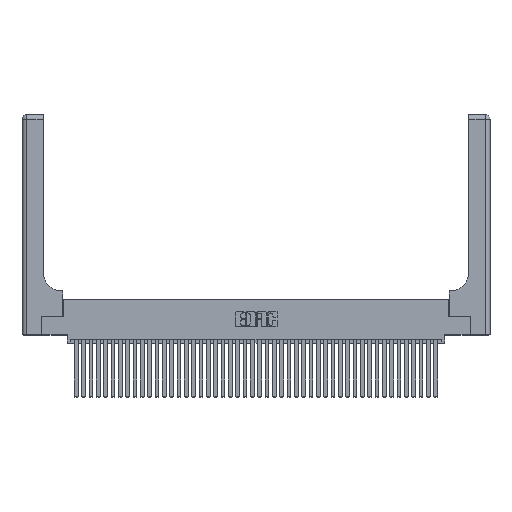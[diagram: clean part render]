
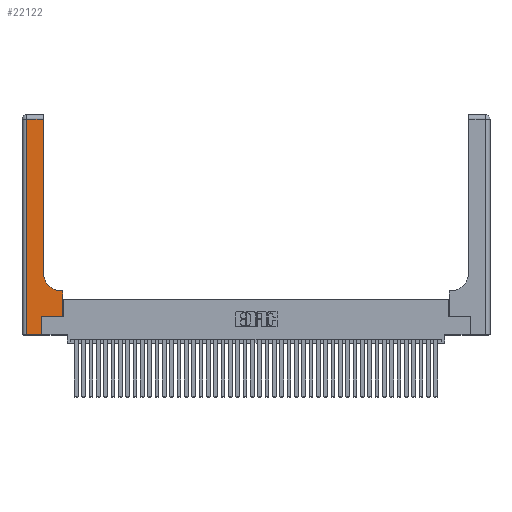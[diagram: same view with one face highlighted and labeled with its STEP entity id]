
A CAD part, top view. The second image highlights one B-rep face of the part: STEP entity #22122.
In plain terms, the highlighted planar face has unit normal (0, 0, 1).
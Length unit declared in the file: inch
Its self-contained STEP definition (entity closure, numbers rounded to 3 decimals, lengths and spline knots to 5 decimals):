
#1675 = ORIENTED_EDGE ( 'NONE', *, *, #29388, .T. ) ;
#1790 = CARTESIAN_POINT ( 'NONE',  ( 0., 2.94, 0.37 ) ) ;
#1828 = VECTOR ( 'NONE', #29314, 39.37008 ) ;
#2134 = ORIENTED_EDGE ( 'NONE', *, *, #26570, .T. ) ;
#2273 = CARTESIAN_POINT ( 'NONE',  ( 0.269, 0., 0.37 ) ) ;
#3231 = CARTESIAN_POINT ( 'NONE',  ( 0.5415, 0.85, 0.37 ) ) ;
#4687 = CARTESIAN_POINT ( 'NONE',  ( 0., 3., 0.37 ) ) ;
#4764 = VECTOR ( 'NONE', #25239, 39.37008 ) ;
#5021 = ORIENTED_EDGE ( 'NONE', *, *, #32963, .T. ) ;
#5341 = LINE ( 'NONE', #16382, #13218 ) ;
#5788 = VECTOR ( 'NONE', #25707, 39.37008 ) ;
#6690 = DIRECTION ( 'NONE',  ( 1., 0., 0. ) ) ;
#6792 = CARTESIAN_POINT ( 'NONE',  ( 0.5585, 0.25, 0.37 ) ) ;
#7036 = EDGE_CURVE ( 'NONE', #40032, #33481, #38440, .T. ) ;
#7800 = FACE_OUTER_BOUND ( 'NONE', #28808, .T. ) ;
#8131 = DIRECTION ( 'NONE',  ( -1., 0., 0. ) ) ;
#10428 = VERTEX_POINT ( 'NONE', #27369 ) ;
#12899 = VERTEX_POINT ( 'NONE', #33126 ) ;
#13218 = VECTOR ( 'NONE', #39647, 39.37008 ) ;
#13805 = VERTEX_POINT ( 'NONE', #41029 ) ;
#13893 = CARTESIAN_POINT ( 'NONE',  ( 0., 0., 0.37 ) ) ;
#14979 = CARTESIAN_POINT ( 'NONE',  ( 0.2915, 3., 0.37 ) ) ;
#16382 = CARTESIAN_POINT ( 'NONE',  ( 0.06, 3., 0.37 ) ) ;
#17123 = EDGE_CURVE ( 'NONE', #33554, #18273, #5341, .T. ) ;
#17316 = EDGE_CURVE ( 'NONE', #18273, #37731, #32512, .T. ) ;
#18273 = VERTEX_POINT ( 'NONE', #21775 ) ;
#19317 = CARTESIAN_POINT ( 'NONE',  ( 0.269, 0., 0.37 ) ) ;
#21311 = DIRECTION ( 'NONE',  ( -1., 0., 0. ) ) ;
#21380 = PLANE ( 'NONE',  #26873 ) ;
#21518 = DIRECTION ( 'NONE',  ( 0., 1., 0. ) ) ;
#21520 = VECTOR ( 'NONE', #21311, 39.37008 ) ;
#21775 = CARTESIAN_POINT ( 'NONE',  ( 0.06, 0., 0.37 ) ) ;
#21965 = CARTESIAN_POINT ( 'NONE',  ( 0.5585, 0.25, 0.37 ) ) ;
#22122 = ADVANCED_FACE ( 'NONE', ( #7800 ), #21380, .F. ) ;
#23458 = CARTESIAN_POINT ( 'NONE',  ( 0.269, 0.25, 0.37 ) ) ;
#23565 = CIRCLE ( 'NONE', #29553, 0.25 ) ;
#23566 = LINE ( 'NONE', #21965, #40195 ) ;
#23633 = VECTOR ( 'NONE', #23931, 39.37008 ) ;
#23657 = ORIENTED_EDGE ( 'NONE', *, *, #17123, .T. ) ;
#23931 = DIRECTION ( 'NONE',  ( 1., 0., 0. ) ) ;
#24382 = LINE ( 'NONE', #14979, #32209 ) ;
#25239 = DIRECTION ( 'NONE',  ( -1., 0., 0. ) ) ;
#25326 = DIRECTION ( 'NONE',  ( 0., 1., 0. ) ) ;
#25707 = DIRECTION ( 'NONE',  ( 0., 1., 0. ) ) ;
#26570 = EDGE_CURVE ( 'NONE', #33481, #13805, #23566, .T. ) ;
#26661 = DIRECTION ( 'NONE',  ( 0., 0., -1. ) ) ;
#26873 = AXIS2_PLACEMENT_3D ( 'NONE', #4687, #28098, #8131 ) ;
#27369 = CARTESIAN_POINT ( 'NONE',  ( 0.2915, 2.94, 0.37 ) ) ;
#27762 = ORIENTED_EDGE ( 'NONE', *, *, #7036, .T. ) ;
#28098 = DIRECTION ( 'NONE',  ( 0., 0., -1. ) ) ;
#28808 = EDGE_LOOP ( 'NONE', ( #5021, #30666, #23657, #37306, #38228, #27762, #2134, #1675, #29925 ) ) ;
#29314 = DIRECTION ( 'NONE',  ( 1., 0., 0. ) ) ;
#29388 = EDGE_CURVE ( 'NONE', #13805, #12899, #40235, .T. ) ;
#29553 = AXIS2_PLACEMENT_3D ( 'NONE', #3231, #26661, #6690 ) ;
#29767 = EDGE_CURVE ( 'NONE', #12899, #37342, #23565, .T. ) ;
#29925 = ORIENTED_EDGE ( 'NONE', *, *, #29767, .T. ) ;
#30390 = LINE ( 'NONE', #1790, #4764 ) ;
#30666 = ORIENTED_EDGE ( 'NONE', *, *, #43251, .T. ) ;
#30836 = CARTESIAN_POINT ( 'NONE',  ( 0.2915, 0.85, 0.37 ) ) ;
#32209 = VECTOR ( 'NONE', #21518, 39.37008 ) ;
#32512 = LINE ( 'NONE', #13893, #23633 ) ;
#32535 = CARTESIAN_POINT ( 'NONE',  ( 0.269, 0.25, 0.37 ) ) ;
#32963 = EDGE_CURVE ( 'NONE', #37342, #10428, #24382, .T. ) ;
#33126 = CARTESIAN_POINT ( 'NONE',  ( 0.5415, 0.6, 0.37 ) ) ;
#33481 = VERTEX_POINT ( 'NONE', #6792 ) ;
#33554 = VERTEX_POINT ( 'NONE', #40258 ) ;
#34560 = CARTESIAN_POINT ( 'NONE',  ( 0.2915, 0.6, 0.37 ) ) ;
#37306 = ORIENTED_EDGE ( 'NONE', *, *, #17316, .T. ) ;
#37342 = VERTEX_POINT ( 'NONE', #30836 ) ;
#37689 = EDGE_CURVE ( 'NONE', #37731, #40032, #39168, .T. ) ;
#37731 = VERTEX_POINT ( 'NONE', #19317 ) ;
#38228 = ORIENTED_EDGE ( 'NONE', *, *, #37689, .T. ) ;
#38440 = LINE ( 'NONE', #32535, #1828 ) ;
#39168 = LINE ( 'NONE', #2273, #5788 ) ;
#39647 = DIRECTION ( 'NONE',  ( 0., -1., 0. ) ) ;
#40032 = VERTEX_POINT ( 'NONE', #23458 ) ;
#40195 = VECTOR ( 'NONE', #25326, 39.37008 ) ;
#40235 = LINE ( 'NONE', #34560, #21520 ) ;
#40258 = CARTESIAN_POINT ( 'NONE',  ( 0.06, 2.94, 0.37 ) ) ;
#41029 = CARTESIAN_POINT ( 'NONE',  ( 0.5585, 0.6, 0.37 ) ) ;
#43251 = EDGE_CURVE ( 'NONE', #10428, #33554, #30390, .T. ) ;
